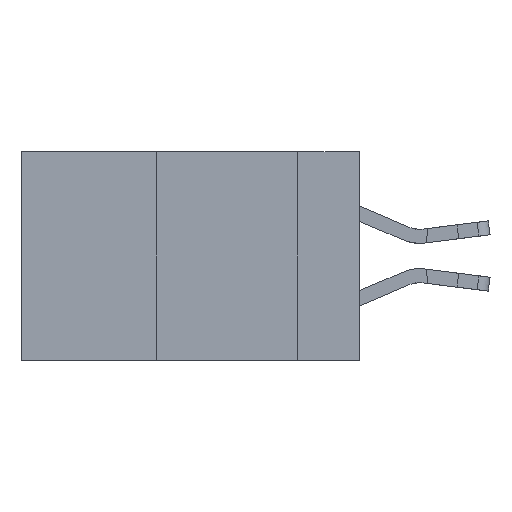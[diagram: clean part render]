
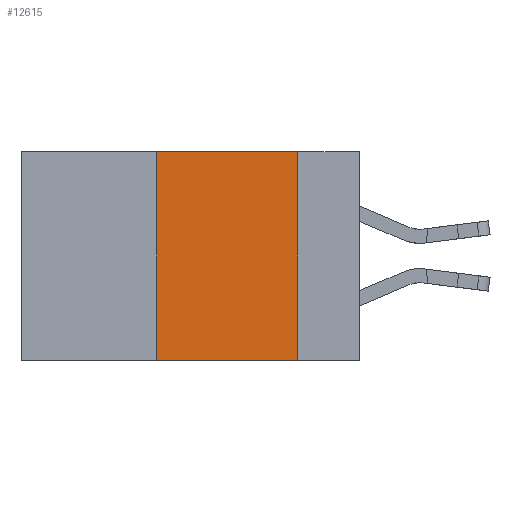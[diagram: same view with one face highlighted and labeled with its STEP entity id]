
A CAD part, left-side view. The second image highlights one B-rep face of the part: STEP entity #12615.
In plain terms, the highlighted planar face has unit normal (-1, 0, 0).
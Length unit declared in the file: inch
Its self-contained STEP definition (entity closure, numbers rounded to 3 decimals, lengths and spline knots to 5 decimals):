
#2186 = DIRECTION ( 'NONE',  ( 0., -1., 0. ) ) ;
#3484 = FACE_OUTER_BOUND ( 'NONE', #9900, .T. ) ;
#3552 = EDGE_CURVE ( 'NONE', #26622, #18553, #33972, .T. ) ;
#4231 = VECTOR ( 'NONE', #35452, 39.37008 ) ;
#5663 = VERTEX_POINT ( 'NONE', #35794 ) ;
#7409 = LINE ( 'NONE', #14149, #25700 ) ;
#9472 = CARTESIAN_POINT ( 'NONE',  ( 0., 0.6, 0. ) ) ;
#9900 = EDGE_LOOP ( 'NONE', ( #20570, #14258, #29187, #25195 ) ) ;
#10406 = LINE ( 'NONE', #35573, #4231 ) ;
#10671 = EDGE_CURVE ( 'NONE', #17943, #5663, #33677, .T. ) ;
#11660 = DIRECTION ( 'NONE',  ( 1., 0., 0. ) ) ;
#12615 = ADVANCED_FACE ( 'NONE', ( #3484 ), #23340, .F. ) ;
#13775 = DIRECTION ( 'NONE',  ( 0., -1., 0. ) ) ;
#14149 = CARTESIAN_POINT ( 'NONE',  ( 0., 0.36, 0. ) ) ;
#14258 = ORIENTED_EDGE ( 'NONE', *, *, #3552, .F. ) ;
#15847 = CARTESIAN_POINT ( 'NONE',  ( 0., 0.11, 0. ) ) ;
#17943 = VERTEX_POINT ( 'NONE', #24876 ) ;
#18553 = VERTEX_POINT ( 'NONE', #15847 ) ;
#19873 = EDGE_CURVE ( 'NONE', #18553, #5663, #10406, .T. ) ;
#20570 = ORIENTED_EDGE ( 'NONE', *, *, #19873, .F. ) ;
#21456 = AXIS2_PLACEMENT_3D ( 'NONE', #9472, #11660, #31072 ) ;
#23340 = PLANE ( 'NONE',  #21456 ) ;
#24357 = CARTESIAN_POINT ( 'NONE',  ( 0., 0.6, 0. ) ) ;
#24836 = CARTESIAN_POINT ( 'NONE',  ( 0., 0.6, -0.37 ) ) ;
#24876 = CARTESIAN_POINT ( 'NONE',  ( 0., 0.36, -0.37 ) ) ;
#25195 = ORIENTED_EDGE ( 'NONE', *, *, #10671, .T. ) ;
#25434 = VECTOR ( 'NONE', #13775, 39.37008 ) ;
#25700 = VECTOR ( 'NONE', #33445, 39.37008 ) ;
#26622 = VERTEX_POINT ( 'NONE', #32754 ) ;
#28985 = EDGE_CURVE ( 'NONE', #17943, #26622, #7409, .T. ) ;
#29187 = ORIENTED_EDGE ( 'NONE', *, *, #28985, .F. ) ;
#30479 = VECTOR ( 'NONE', #2186, 39.37008 ) ;
#31072 = DIRECTION ( 'NONE',  ( 0., 0., -1. ) ) ;
#32754 = CARTESIAN_POINT ( 'NONE',  ( 0., 0.36, 0. ) ) ;
#33445 = DIRECTION ( 'NONE',  ( 0., 0., 1. ) ) ;
#33677 = LINE ( 'NONE', #24836, #25434 ) ;
#33972 = LINE ( 'NONE', #24357, #30479 ) ;
#35452 = DIRECTION ( 'NONE',  ( 0., 0., -1. ) ) ;
#35573 = CARTESIAN_POINT ( 'NONE',  ( 0., 0.11, 0. ) ) ;
#35794 = CARTESIAN_POINT ( 'NONE',  ( 0., 0.11, -0.37 ) ) ;
